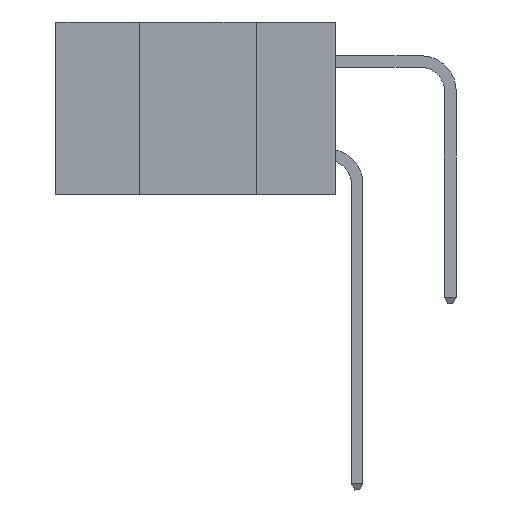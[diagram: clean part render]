
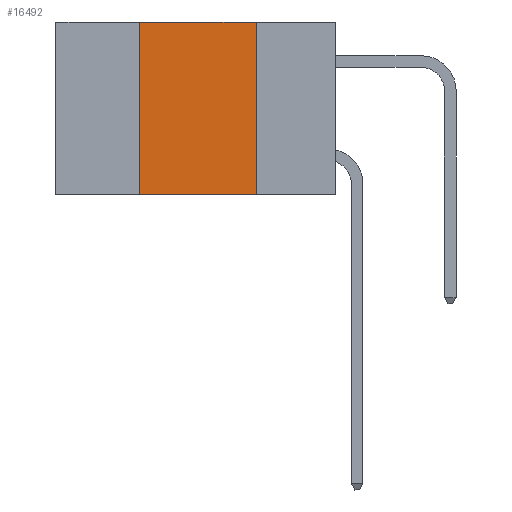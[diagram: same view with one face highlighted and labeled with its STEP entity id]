
A CAD part, left-side view. The second image highlights one B-rep face of the part: STEP entity #16492.
In plain terms, the highlighted planar face has unit normal (-1, 0, 0).
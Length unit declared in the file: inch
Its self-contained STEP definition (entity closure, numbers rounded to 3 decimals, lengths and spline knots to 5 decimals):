
#105 = CARTESIAN_POINT ( 'NONE',  ( 0., 0.42, 0. ) ) ;
#538 = DIRECTION ( 'NONE',  ( 0., -1., 0. ) ) ;
#1329 = CARTESIAN_POINT ( 'NONE',  ( 0., 0.6, 0. ) ) ;
#1507 = CARTESIAN_POINT ( 'NONE',  ( 0., 0.17, -0.37 ) ) ;
#1765 = VECTOR ( 'NONE', #16016, 39.37008 ) ;
#3246 = LINE ( 'NONE', #30532, #27792 ) ;
#3726 = DIRECTION ( 'NONE',  ( 0., 0., -1. ) ) ;
#4148 = DIRECTION ( 'NONE',  ( 0., -1., 0. ) ) ;
#5989 = ORIENTED_EDGE ( 'NONE', *, *, #29756, .T. ) ;
#6212 = AXIS2_PLACEMENT_3D ( 'NONE', #1329, #18051, #11314 ) ;
#8407 = VERTEX_POINT ( 'NONE', #1507 ) ;
#8493 = ORIENTED_EDGE ( 'NONE', *, *, #27712, .F. ) ;
#11199 = ORIENTED_EDGE ( 'NONE', *, *, #17515, .F. ) ;
#11314 = DIRECTION ( 'NONE',  ( 0., 0., -1. ) ) ;
#12223 = LINE ( 'NONE', #22903, #30391 ) ;
#13405 = VERTEX_POINT ( 'NONE', #21999 ) ;
#15091 = VERTEX_POINT ( 'NONE', #105 ) ;
#16016 = DIRECTION ( 'NONE',  ( 0., 0., 1. ) ) ;
#16492 = ADVANCED_FACE ( 'NONE', ( #18946 ), #17240, .F. ) ;
#17240 = PLANE ( 'NONE',  #6212 ) ;
#17515 = EDGE_CURVE ( 'NONE', #15091, #13405, #3246, .T. ) ;
#18051 = DIRECTION ( 'NONE',  ( 1., 0., 0. ) ) ;
#18462 = EDGE_LOOP ( 'NONE', ( #8493, #11199, #21088, #5989 ) ) ;
#18946 = FACE_OUTER_BOUND ( 'NONE', #18462, .T. ) ;
#19884 = VECTOR ( 'NONE', #538, 39.37008 ) ;
#20624 = LINE ( 'NONE', #20626, #19884 ) ;
#20626 = CARTESIAN_POINT ( 'NONE',  ( 0., 0.6, -0.37 ) ) ;
#21088 = ORIENTED_EDGE ( 'NONE', *, *, #27763, .F. ) ;
#21999 = CARTESIAN_POINT ( 'NONE',  ( 0., 0.17, 0. ) ) ;
#22266 = CARTESIAN_POINT ( 'NONE',  ( 0., 0.42, -0.37 ) ) ;
#22903 = CARTESIAN_POINT ( 'NONE',  ( 0., 0.17, 0. ) ) ;
#24858 = LINE ( 'NONE', #27839, #1765 ) ;
#27712 = EDGE_CURVE ( 'NONE', #13405, #8407, #12223, .T. ) ;
#27763 = EDGE_CURVE ( 'NONE', #28382, #15091, #24858, .T. ) ;
#27792 = VECTOR ( 'NONE', #4148, 39.37008 ) ;
#27839 = CARTESIAN_POINT ( 'NONE',  ( 0., 0.42, 0. ) ) ;
#28382 = VERTEX_POINT ( 'NONE', #22266 ) ;
#29756 = EDGE_CURVE ( 'NONE', #28382, #8407, #20624, .T. ) ;
#30391 = VECTOR ( 'NONE', #3726, 39.37008 ) ;
#30532 = CARTESIAN_POINT ( 'NONE',  ( 0., 0.6, 0. ) ) ;
